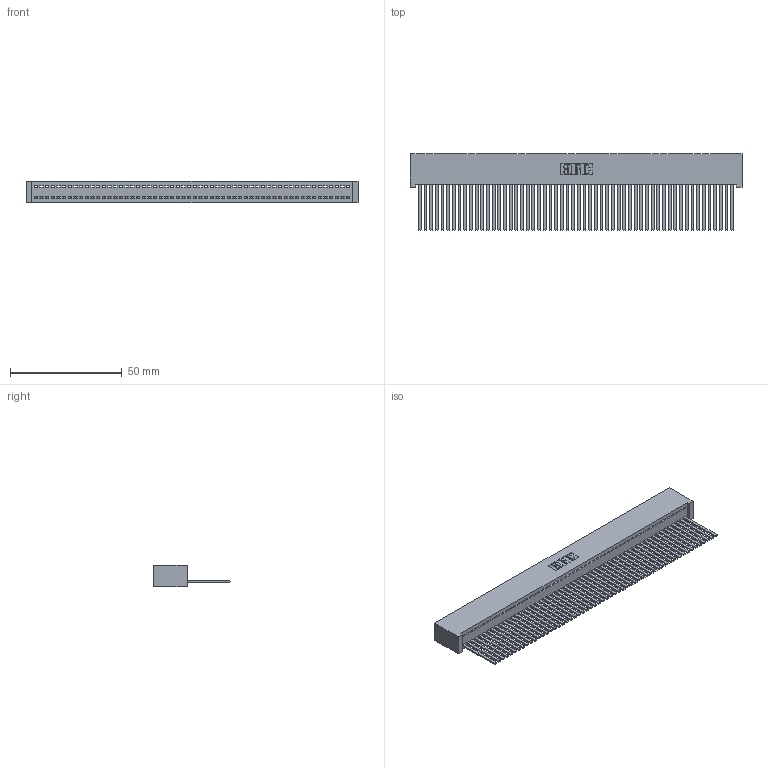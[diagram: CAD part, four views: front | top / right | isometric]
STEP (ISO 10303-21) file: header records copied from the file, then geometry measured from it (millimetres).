
FILE_DESCRIPTION (( 'STEP AP203' ), '1' );
FILE_NAME ('392-056-544-101.STEP', '2019-10-08T15:18:15', ( '' ), ( '' ), 'SwSTEP 2.0', 'SolidWorks 2016', '' );
FILE_SCHEMA (( 'CONFIG_CONTROL_DESIGN' ));
Length unit declared in the file: inch
Products named in the file (3): 342 Part_Lugless; 345-292-001_345-293-144; 392-056-544-101
Assembly tree (57 placements, depth 2):
  392-056-544-101
    342 Part_Lugless
    345-292-001_345-293-144  x56
Bounding box: 148.49 x 34.3 x 9.4 mm (x, y, z)
Volume: 14128.6 mm3; surface area: 23177.7 mm2
Topology: 57 solids, 57 shells, 3014 faces, 9123 edges, 6006 vertices
Faces by surface type: plane 2190, cylinder 824
Entity records: 31831 total; most frequent: CARTESIAN_POINT 5494, ORIENTED_EDGE 5486, DIRECTION 4595, EDGE_CURVE 2743, VECTOR 2627, LINE 2627, VERTEX_POINT 1826, AXIS2_PLACEMENT_3D 984
